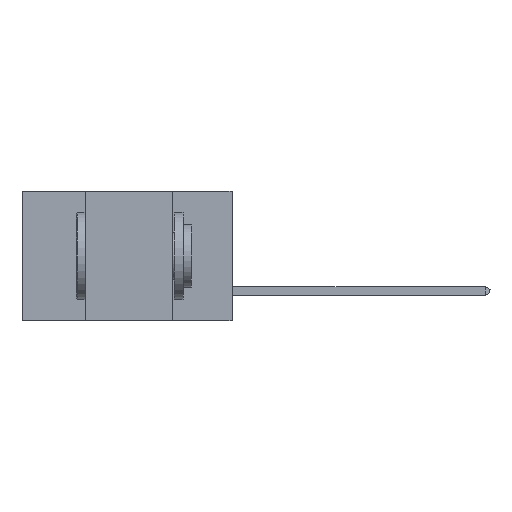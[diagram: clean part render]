
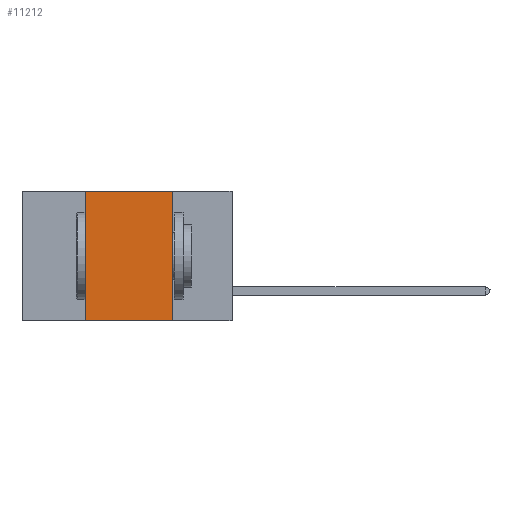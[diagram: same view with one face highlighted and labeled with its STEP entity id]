
A CAD part, left-side view. The second image highlights one B-rep face of the part: STEP entity #11212.
In plain terms, the highlighted planar face has unit normal (-1, 0, 0).
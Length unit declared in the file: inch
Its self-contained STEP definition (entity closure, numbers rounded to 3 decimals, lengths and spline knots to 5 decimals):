
#562 = VECTOR ( 'NONE', #4247, 39.37008 ) ;
#2047 = EDGE_CURVE ( 'NONE', #7441, #7469, #23595, .T. ) ;
#2170 = LINE ( 'NONE', #6318, #17949 ) ;
#2757 = ORIENTED_EDGE ( 'NONE', *, *, #16331, .F. ) ;
#4247 = DIRECTION ( 'NONE',  ( 0., 0., 1. ) ) ;
#5538 = ORIENTED_EDGE ( 'NONE', *, *, #2047, .F. ) ;
#6318 = CARTESIAN_POINT ( 'NONE',  ( 0., 0.6, -0.37 ) ) ;
#7049 = LINE ( 'NONE', #11553, #562 ) ;
#7200 = DIRECTION ( 'NONE',  ( 0., -1., 0. ) ) ;
#7283 = DIRECTION ( 'NONE',  ( 0., 0., -1. ) ) ;
#7441 = VERTEX_POINT ( 'NONE', #10914 ) ;
#7469 = VERTEX_POINT ( 'NONE', #14783 ) ;
#8161 = LINE ( 'NONE', #20216, #11990 ) ;
#8959 = DIRECTION ( 'NONE',  ( 1., 0., 0. ) ) ;
#10914 = CARTESIAN_POINT ( 'NONE',  ( 0., 0.17, 0. ) ) ;
#11212 = ADVANCED_FACE ( 'NONE', ( #14023 ), #16682, .F. ) ;
#11553 = CARTESIAN_POINT ( 'NONE',  ( 0., 0.42, 0. ) ) ;
#11987 = DIRECTION ( 'NONE',  ( 0., -1., 0. ) ) ;
#11990 = VECTOR ( 'NONE', #7200, 39.37008 ) ;
#12155 = AXIS2_PLACEMENT_3D ( 'NONE', #20221, #8959, #7283 ) ;
#13676 = CARTESIAN_POINT ( 'NONE',  ( 0., 0.42, 0. ) ) ;
#14023 = FACE_OUTER_BOUND ( 'NONE', #17181, .T. ) ;
#14419 = ORIENTED_EDGE ( 'NONE', *, *, #21212, .T. ) ;
#14625 = CARTESIAN_POINT ( 'NONE',  ( 0., 0.42, -0.37 ) ) ;
#14783 = CARTESIAN_POINT ( 'NONE',  ( 0., 0.17, -0.37 ) ) ;
#15248 = CARTESIAN_POINT ( 'NONE',  ( 0., 0.17, 0. ) ) ;
#16331 = EDGE_CURVE ( 'NONE', #20945, #18708, #7049, .T. ) ;
#16682 = PLANE ( 'NONE',  #12155 ) ;
#17031 = DIRECTION ( 'NONE',  ( 0., 0., -1. ) ) ;
#17181 = EDGE_LOOP ( 'NONE', ( #5538, #17378, #2757, #14419 ) ) ;
#17378 = ORIENTED_EDGE ( 'NONE', *, *, #20594, .F. ) ;
#17949 = VECTOR ( 'NONE', #11987, 39.37008 ) ;
#18708 = VERTEX_POINT ( 'NONE', #13676 ) ;
#19808 = VECTOR ( 'NONE', #17031, 39.37008 ) ;
#20216 = CARTESIAN_POINT ( 'NONE',  ( 0., 0.6, 0. ) ) ;
#20221 = CARTESIAN_POINT ( 'NONE',  ( 0., 0.6, 0. ) ) ;
#20594 = EDGE_CURVE ( 'NONE', #18708, #7441, #8161, .T. ) ;
#20945 = VERTEX_POINT ( 'NONE', #14625 ) ;
#21212 = EDGE_CURVE ( 'NONE', #20945, #7469, #2170, .T. ) ;
#23595 = LINE ( 'NONE', #15248, #19808 ) ;
